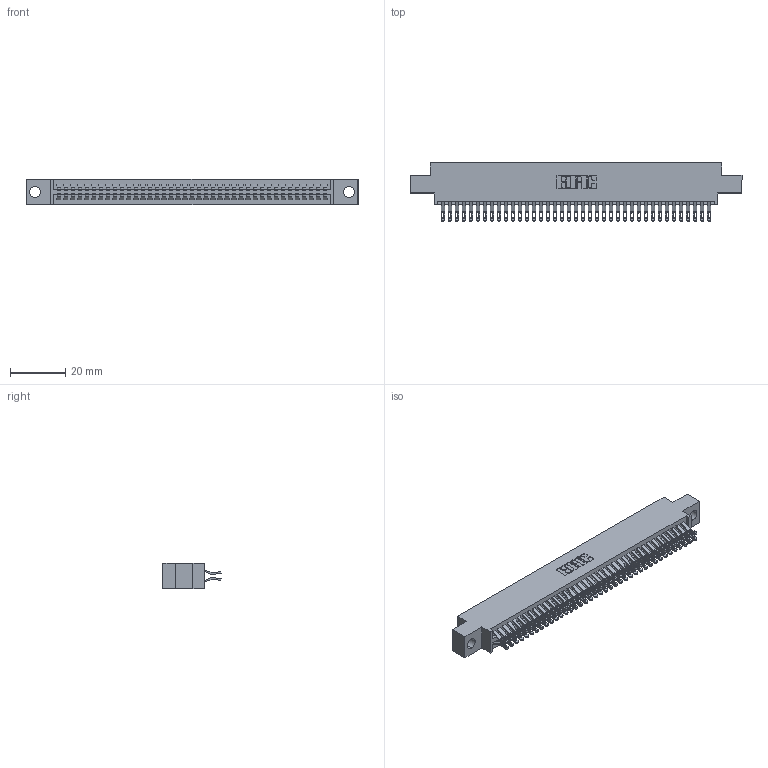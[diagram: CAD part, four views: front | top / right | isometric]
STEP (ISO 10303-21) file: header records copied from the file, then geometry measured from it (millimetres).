
FILE_DESCRIPTION (( 'STEP AP203' ), '1' );
FILE_NAME ('395-078-555-804.STEP', '2018-11-28T01:29:30', ( '' ), ( '' ), 'SwSTEP 2.0', 'SolidWorks 2016', '' );
FILE_SCHEMA (( 'CONFIG_CONTROL_DESIGN' ));
Length unit declared in the file: inch
Products named in the file (3): 345 Part_0.170 Offset - 0.156 Dia-TH; 395-078-555-804; 345-292-001_555 Tail
Assembly tree (79 placements, depth 2):
  395-078-555-804
    345 Part_0.170 Offset - 0.156 Dia-TH
    345-292-001_555 Tail  x78
Bounding box: 120.27 x 21.13 x 9.4 mm (x, y, z)
Volume: 11680.2 mm3; surface area: 17952.8 mm2
Topology: 79 solids, 79 shells, 4498 faces, 14159 edges, 9438 vertices
Faces by surface type: plane 2502, cylinder 1996
Entity records: 31465 total; most frequent: CARTESIAN_POINT 5314, ORIENTED_EDGE 5218, DIRECTION 4657, EDGE_CURVE 2609, LINE 2301, VECTOR 2301, VERTEX_POINT 1738, AXIS2_PLACEMENT_3D 1178
